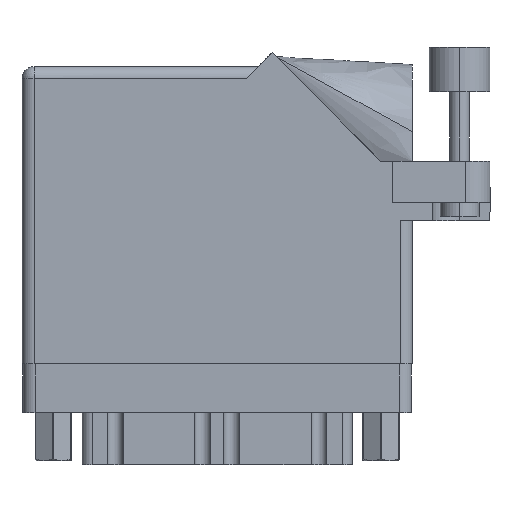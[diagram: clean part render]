
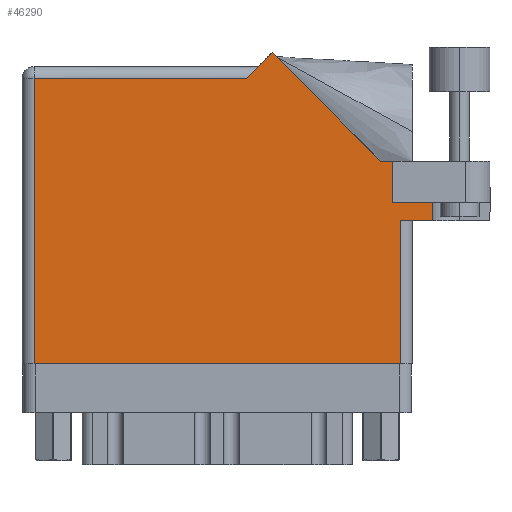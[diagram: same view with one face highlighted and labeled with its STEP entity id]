
A CAD part, front view. The second image highlights one B-rep face of the part: STEP entity #46290.
In plain terms, the highlighted face is planar.
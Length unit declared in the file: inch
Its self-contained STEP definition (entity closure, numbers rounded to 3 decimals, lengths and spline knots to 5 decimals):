
#391 = VERTEX_POINT ( 'NONE', #30574 ) ;
#519 = ORIENTED_EDGE ( 'NONE', *, *, #8042, .F. ) ;
#1669 = EDGE_CURVE ( 'NONE', #34116, #35301, #43491, .T. ) ;
#1953 = LINE ( 'NONE', #35568, #47797 ) ;
#2954 = LINE ( 'NONE', #24979, #43916 ) ;
#3286 = DIRECTION ( 'NONE',  ( 0., 0., -1. ) ) ;
#4063 = CARTESIAN_POINT ( 'NONE',  ( 0.062, 0., 0. ) ) ;
#4414 = VECTOR ( 'NONE', #39880, 39.37008 ) ;
#4901 = CARTESIAN_POINT ( 'NONE',  ( 2.01, 0.737, 0. ) ) ;
#4992 = DIRECTION ( 'NONE',  ( 1., 0., 0. ) ) ;
#5737 = VECTOR ( 'NONE', #45717, 39.37008 ) ;
#6636 = VECTOR ( 'NONE', #4992, 39.37008 ) ;
#8042 = EDGE_CURVE ( 'NONE', #36723, #391, #24899, .T. ) ;
#8279 = CARTESIAN_POINT ( 'NONE',  ( 1.91, 1.044, 0. ) ) ;
#8623 = CARTESIAN_POINT ( 'NONE',  ( 0., 0., 0. ) ) ;
#9270 = ORIENTED_EDGE ( 'NONE', *, *, #19804, .T. ) ;
#9409 = ORIENTED_EDGE ( 'NONE', *, *, #23947, .F. ) ;
#10144 = CARTESIAN_POINT ( 'NONE',  ( 2.1115, 1.16177, 0. ) ) ;
#10468 = EDGE_CURVE ( 'NONE', #13535, #36226, #44310, .T. ) ;
#11490 = CARTESIAN_POINT ( 'NONE',  ( 2.1115, 0.831, 0. ) ) ;
#11591 = EDGE_CURVE ( 'NONE', #27808, #13535, #17246, .T. ) ;
#12613 = CARTESIAN_POINT ( 'NONE',  ( 0.062, 1.468, 0. ) ) ;
#12757 = EDGE_CURVE ( 'NONE', #33104, #27808, #23446, .T. ) ;
#13443 = LINE ( 'NONE', #8623, #6636 ) ;
#13535 = VERTEX_POINT ( 'NONE', #12613 ) ;
#14801 = VERTEX_POINT ( 'NONE', #29418 ) ;
#15227 = VECTOR ( 'NONE', #35626, 39.37008 ) ;
#15400 = CARTESIAN_POINT ( 'NONE',  ( 1.84442, 1.044, 0. ) ) ;
#16348 = CARTESIAN_POINT ( 'NONE',  ( 0., 1.468, 0. ) ) ;
#16385 = VERTEX_POINT ( 'NONE', #46254 ) ;
#16927 = ORIENTED_EDGE ( 'NONE', *, *, #11591, .T. ) ;
#17246 = LINE ( 'NONE', #16348, #15227 ) ;
#19585 = VECTOR ( 'NONE', #23837, 39.37008 ) ;
#19804 = EDGE_CURVE ( 'NONE', #14801, #44306, #2954, .T. ) ;
#20208 = LINE ( 'NONE', #27454, #19585 ) ;
#20926 = ORIENTED_EDGE ( 'NONE', *, *, #10468, .T. ) ;
#21534 = VECTOR ( 'NONE', #40703, 39.37008 ) ;
#22418 = ORIENTED_EDGE ( 'NONE', *, *, #35534, .T. ) ;
#22609 = FACE_OUTER_BOUND ( 'NONE', #29562, .T. ) ;
#22864 = VECTOR ( 'NONE', #36001, 39.37008 ) ;
#23446 = LINE ( 'NONE', #38172, #30733 ) ;
#23837 = DIRECTION ( 'NONE',  ( 0., 1., 0. ) ) ;
#23947 = EDGE_CURVE ( 'NONE', #16385, #36723, #1953, .T. ) ;
#23976 = DIRECTION ( 'NONE',  ( 1., 0., 0. ) ) ;
#24218 = LINE ( 'NONE', #28812, #44786 ) ;
#24899 = LINE ( 'NONE', #10144, #22864 ) ;
#24979 = CARTESIAN_POINT ( 'NONE',  ( 1.948, 0.737, 0. ) ) ;
#25335 = EDGE_CURVE ( 'NONE', #35301, #33104, #24218, .T. ) ;
#27454 = CARTESIAN_POINT ( 'NONE',  ( 1.91, 0.831, 0. ) ) ;
#27808 = VERTEX_POINT ( 'NONE', #35648 ) ;
#28145 = ORIENTED_EDGE ( 'NONE', *, *, #40842, .T. ) ;
#28478 = ORIENTED_EDGE ( 'NONE', *, *, #1669, .T. ) ;
#28665 = CARTESIAN_POINT ( 'NONE',  ( 0.062, 0., 0. ) ) ;
#28812 = CARTESIAN_POINT ( 'NONE',  ( 1.84442, 1.044, 0. ) ) ;
#29418 = CARTESIAN_POINT ( 'NONE',  ( 1.948, 0., 0. ) ) ;
#29562 = EDGE_LOOP ( 'NONE', ( #22418, #9270, #35762, #519, #9409, #28145, #28478, #31456, #36145, #16927, #20926 ) ) ;
#29987 = DIRECTION ( 'NONE',  ( -0.707, -0.707, 0. ) ) ;
#30191 = DIRECTION ( 'NONE',  ( 0., 1., 0. ) ) ;
#30574 = CARTESIAN_POINT ( 'NONE',  ( 2.1115, 0.737, 0. ) ) ;
#30733 = VECTOR ( 'NONE', #29987, 39.37008 ) ;
#31456 = ORIENTED_EDGE ( 'NONE', *, *, #25335, .T. ) ;
#32402 = CARTESIAN_POINT ( 'NONE',  ( 1.948, 0.737, 0. ) ) ;
#32637 = CARTESIAN_POINT ( 'NONE',  ( 2.41, 1.044, 0. ) ) ;
#33104 = VERTEX_POINT ( 'NONE', #44112 ) ;
#34116 = VERTEX_POINT ( 'NONE', #8279 ) ;
#34617 = LINE ( 'NONE', #4901, #5737 ) ;
#35301 = VERTEX_POINT ( 'NONE', #15400 ) ;
#35534 = EDGE_CURVE ( 'NONE', #36226, #14801, #13443, .T. ) ;
#35568 = CARTESIAN_POINT ( 'NONE',  ( 1.91, 0.831, 0. ) ) ;
#35626 = DIRECTION ( 'NONE',  ( -1., 0., 0. ) ) ;
#35648 = CARTESIAN_POINT ( 'NONE',  ( 1.155, 1.468, 0. ) ) ;
#35762 = ORIENTED_EDGE ( 'NONE', *, *, #37313, .T. ) ;
#36001 = DIRECTION ( 'NONE',  ( 0., -1., 0. ) ) ;
#36145 = ORIENTED_EDGE ( 'NONE', *, *, #12757, .T. ) ;
#36226 = VERTEX_POINT ( 'NONE', #4063 ) ;
#36408 = PLANE ( 'NONE',  #39584 ) ;
#36723 = VERTEX_POINT ( 'NONE', #11490 ) ;
#37313 = EDGE_CURVE ( 'NONE', #44306, #391, #34617, .T. ) ;
#38172 = CARTESIAN_POINT ( 'NONE',  ( 1.217, 1.53, 0. ) ) ;
#39584 = AXIS2_PLACEMENT_3D ( 'NONE', #44562, #3286, #47489 ) ;
#39880 = DIRECTION ( 'NONE',  ( -1., 0., 0. ) ) ;
#40703 = DIRECTION ( 'NONE',  ( 0., -1., 0. ) ) ;
#40842 = EDGE_CURVE ( 'NONE', #16385, #34116, #20208, .T. ) ;
#42798 = DIRECTION ( 'NONE',  ( -0.707, 0.707, 0. ) ) ;
#43491 = LINE ( 'NONE', #32637, #4414 ) ;
#43916 = VECTOR ( 'NONE', #30191, 39.37008 ) ;
#44112 = CARTESIAN_POINT ( 'NONE',  ( 1.28771, 1.60071, 0. ) ) ;
#44306 = VERTEX_POINT ( 'NONE', #32402 ) ;
#44310 = LINE ( 'NONE', #28665, #21534 ) ;
#44562 = CARTESIAN_POINT ( 'NONE',  ( 0., 1.53, 0. ) ) ;
#44786 = VECTOR ( 'NONE', #42798, 39.37008 ) ;
#45717 = DIRECTION ( 'NONE',  ( 1., 0., 0. ) ) ;
#46254 = CARTESIAN_POINT ( 'NONE',  ( 1.91, 0.831, 0. ) ) ;
#46290 = ADVANCED_FACE ( 'NONE', ( #22609 ), #36408, .F. ) ;
#47489 = DIRECTION ( 'NONE',  ( -1., 0., 0. ) ) ;
#47797 = VECTOR ( 'NONE', #23976, 39.37008 ) ;
